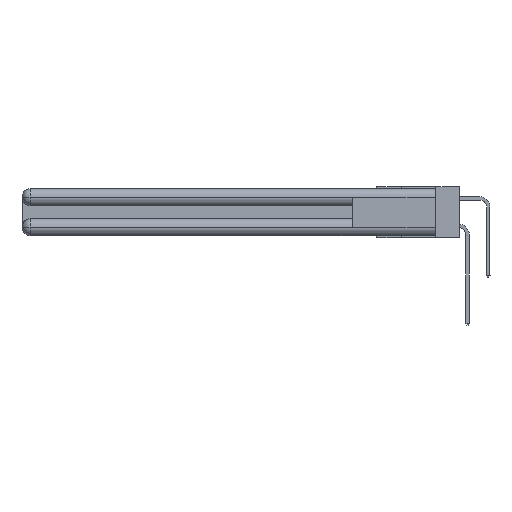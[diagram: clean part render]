
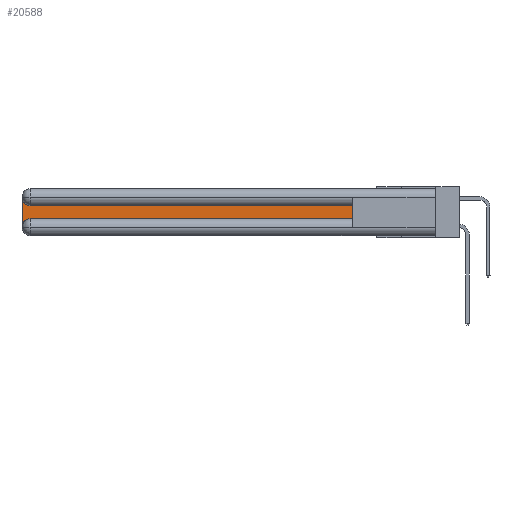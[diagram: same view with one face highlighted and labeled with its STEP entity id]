
A CAD part, left-side view. The second image highlights one B-rep face of the part: STEP entity #20588.
In plain terms, the highlighted planar face has unit normal (-1, 0, 0).
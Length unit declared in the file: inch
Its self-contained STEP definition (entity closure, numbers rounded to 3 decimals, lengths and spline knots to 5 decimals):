
#430 = DIRECTION ( 'NONE',  ( 0., 0., 1. ) ) ;
#1101 = EDGE_CURVE ( 'NONE', #32947, #29765, #9955, .T. ) ;
#2810 = CARTESIAN_POINT ( 'NONE',  ( 0.075, 2.94, -0.2775 ) ) ;
#3020 = CARTESIAN_POINT ( 'NONE',  ( 0.075, 0.6, -0.1225 ) ) ;
#3513 = LINE ( 'NONE', #11790, #24404 ) ;
#3909 = CARTESIAN_POINT ( 'NONE',  ( 0.075, 3., -0.1225 ) ) ;
#3948 = AXIS2_PLACEMENT_3D ( 'NONE', #7678, #23392, #23271 ) ;
#4088 = EDGE_CURVE ( 'NONE', #29081, #18345, #33026, .T. ) ;
#5262 = CARTESIAN_POINT ( 'NONE',  ( 0.075, 3., -0.0625 ) ) ;
#5325 = AXIS2_PLACEMENT_3D ( 'NONE', #2810, #21127, #5445 ) ;
#5445 = DIRECTION ( 'NONE',  ( 0., 0., -1. ) ) ;
#7678 = CARTESIAN_POINT ( 'NONE',  ( 0.075, 2.94, -0.0625 ) ) ;
#7920 = ORIENTED_EDGE ( 'NONE', *, *, #15336, .T. ) ;
#9026 = VECTOR ( 'NONE', #30686, 39.37008 ) ;
#9064 = DIRECTION ( 'NONE',  ( 1., 0., 0. ) ) ;
#9955 = LINE ( 'NONE', #10751, #19788 ) ;
#10751 = CARTESIAN_POINT ( 'NONE',  ( 0.075, 0.6, -0.2175 ) ) ;
#11790 = CARTESIAN_POINT ( 'NONE',  ( 0.075, 0.6, -0.1225 ) ) ;
#12344 = EDGE_LOOP ( 'NONE', ( #27576, #14272, #16632, #26519, #7920, #31642 ) ) ;
#14272 = ORIENTED_EDGE ( 'NONE', *, *, #28520, .T. ) ;
#14622 = DIRECTION ( 'NONE',  ( 0., 1., 0. ) ) ;
#14666 = VERTEX_POINT ( 'NONE', #25025 ) ;
#15336 = EDGE_CURVE ( 'NONE', #31035, #32947, #27049, .T. ) ;
#16632 = ORIENTED_EDGE ( 'NONE', *, *, #4088, .T. ) ;
#18058 = EDGE_CURVE ( 'NONE', #18345, #31035, #18718, .T. ) ;
#18345 = VERTEX_POINT ( 'NONE', #28692 ) ;
#18718 = CIRCLE ( 'NONE', #5325, 0.06 ) ;
#19078 = EDGE_CURVE ( 'NONE', #29765, #14666, #3513, .T. ) ;
#19788 = VECTOR ( 'NONE', #430, 39.37008 ) ;
#20588 = ADVANCED_FACE ( 'NONE', ( #27943 ), #32620, .F. ) ;
#21127 = DIRECTION ( 'NONE',  ( 1., 0., 0. ) ) ;
#22424 = CARTESIAN_POINT ( 'NONE',  ( 0.075, 2.94, -0.2175 ) ) ;
#23271 = DIRECTION ( 'NONE',  ( 0., 0., -1. ) ) ;
#23392 = DIRECTION ( 'NONE',  ( 1., 0., 0. ) ) ;
#23774 = AXIS2_PLACEMENT_3D ( 'NONE', #3909, #9064, #27468 ) ;
#24032 = CARTESIAN_POINT ( 'NONE',  ( 0.075, 3., -0.2175 ) ) ;
#24404 = VECTOR ( 'NONE', #14622, 39.37008 ) ;
#25025 = CARTESIAN_POINT ( 'NONE',  ( 0.075, 2.94, -0.1225 ) ) ;
#26090 = VECTOR ( 'NONE', #28460, 39.37008 ) ;
#26519 = ORIENTED_EDGE ( 'NONE', *, *, #18058, .T. ) ;
#27049 = LINE ( 'NONE', #28279, #9026 ) ;
#27468 = DIRECTION ( 'NONE',  ( 0., 0., -1. ) ) ;
#27576 = ORIENTED_EDGE ( 'NONE', *, *, #19078, .T. ) ;
#27943 = FACE_OUTER_BOUND ( 'NONE', #12344, .T. ) ;
#28279 = CARTESIAN_POINT ( 'NONE',  ( 0.075, 0.6, -0.2175 ) ) ;
#28460 = DIRECTION ( 'NONE',  ( 0., 0., -1. ) ) ;
#28520 = EDGE_CURVE ( 'NONE', #14666, #29081, #29849, .T. ) ;
#28692 = CARTESIAN_POINT ( 'NONE',  ( 0.075, 3., -0.2775 ) ) ;
#29081 = VERTEX_POINT ( 'NONE', #5262 ) ;
#29765 = VERTEX_POINT ( 'NONE', #3020 ) ;
#29849 = CIRCLE ( 'NONE', #3948, 0.06 ) ;
#30686 = DIRECTION ( 'NONE',  ( 0., -1., 0. ) ) ;
#30759 = CARTESIAN_POINT ( 'NONE',  ( 0.075, 0.6, -0.2175 ) ) ;
#31035 = VERTEX_POINT ( 'NONE', #22424 ) ;
#31642 = ORIENTED_EDGE ( 'NONE', *, *, #1101, .T. ) ;
#32620 = PLANE ( 'NONE',  #23774 ) ;
#32947 = VERTEX_POINT ( 'NONE', #30759 ) ;
#33026 = LINE ( 'NONE', #24032, #26090 ) ;
